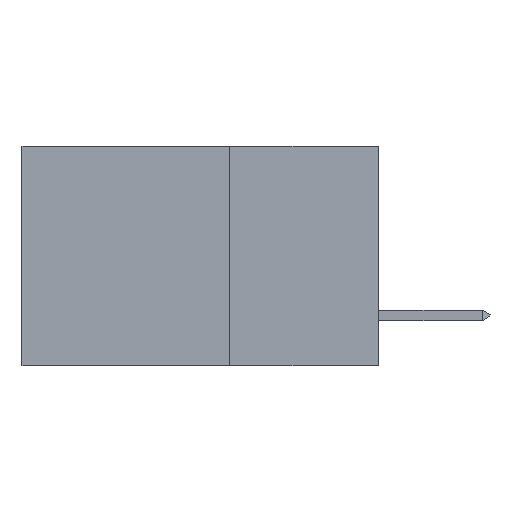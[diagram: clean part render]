
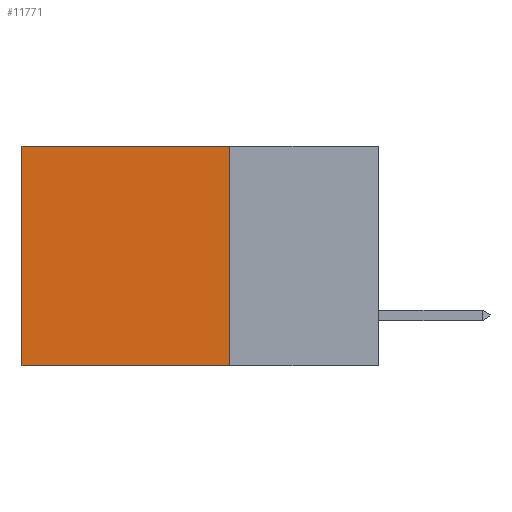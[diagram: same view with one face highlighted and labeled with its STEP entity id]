
A CAD part, left-side view. The second image highlights one B-rep face of the part: STEP entity #11771.
In plain terms, the highlighted planar face has unit normal (-1, 0, 0).
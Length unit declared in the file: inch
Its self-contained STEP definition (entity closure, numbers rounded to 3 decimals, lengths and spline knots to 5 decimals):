
#22 = VECTOR ( 'NONE', #3976, 39.37008 ) ;
#411 = EDGE_CURVE ( 'NONE', #11928, #7889, #801, .T. ) ;
#801 = LINE ( 'NONE', #11834, #3506 ) ;
#879 = EDGE_CURVE ( 'NONE', #6052, #7889, #10992, .T. ) ;
#984 = ORIENTED_EDGE ( 'NONE', *, *, #5597, .F. ) ;
#1007 = ORIENTED_EDGE ( 'NONE', *, *, #5497, .T. ) ;
#1047 = CARTESIAN_POINT ( 'NONE',  ( 0.298, 0.6, 0. ) ) ;
#1145 = DIRECTION ( 'NONE',  ( 0., 0., -1. ) ) ;
#1468 = DIRECTION ( 'NONE',  ( 0., 1., 0. ) ) ;
#1793 = CARTESIAN_POINT ( 'NONE',  ( 0.298, 0.25, 0. ) ) ;
#2299 = CARTESIAN_POINT ( 'NONE',  ( 0.298, 0.25, -0.37 ) ) ;
#3506 = VECTOR ( 'NONE', #1468, 39.37008 ) ;
#3549 = LINE ( 'NONE', #3564, #8967 ) ;
#3564 = CARTESIAN_POINT ( 'NONE',  ( 0.298, 0.25, 0. ) ) ;
#3764 = FACE_OUTER_BOUND ( 'NONE', #10693, .T. ) ;
#3894 = LINE ( 'NONE', #1793, #9603 ) ;
#3976 = DIRECTION ( 'NONE',  ( 0., 0., -1. ) ) ;
#4881 = PLANE ( 'NONE',  #5371 ) ;
#5371 = AXIS2_PLACEMENT_3D ( 'NONE', #9572, #10713, #7845 ) ;
#5497 = EDGE_CURVE ( 'NONE', #9509, #6052, #3549, .T. ) ;
#5597 = EDGE_CURVE ( 'NONE', #9509, #11928, #3894, .T. ) ;
#6052 = VERTEX_POINT ( 'NONE', #6452 ) ;
#6452 = CARTESIAN_POINT ( 'NONE',  ( 0.298, 0.6, 0. ) ) ;
#7845 = DIRECTION ( 'NONE',  ( 0., 0., -1. ) ) ;
#7889 = VERTEX_POINT ( 'NONE', #8202 ) ;
#8202 = CARTESIAN_POINT ( 'NONE',  ( 0.298, 0.6, -0.37 ) ) ;
#8967 = VECTOR ( 'NONE', #9343, 39.37008 ) ;
#9343 = DIRECTION ( 'NONE',  ( 0., 1., 0. ) ) ;
#9509 = VERTEX_POINT ( 'NONE', #9685 ) ;
#9572 = CARTESIAN_POINT ( 'NONE',  ( 0.298, 0.25, 0. ) ) ;
#9603 = VECTOR ( 'NONE', #1145, 39.37008 ) ;
#9683 = ORIENTED_EDGE ( 'NONE', *, *, #411, .F. ) ;
#9685 = CARTESIAN_POINT ( 'NONE',  ( 0.298, 0.25, 0. ) ) ;
#10489 = ORIENTED_EDGE ( 'NONE', *, *, #879, .T. ) ;
#10693 = EDGE_LOOP ( 'NONE', ( #10489, #9683, #984, #1007 ) ) ;
#10713 = DIRECTION ( 'NONE',  ( 1., 0., 0. ) ) ;
#10992 = LINE ( 'NONE', #1047, #22 ) ;
#11771 = ADVANCED_FACE ( 'NONE', ( #3764 ), #4881, .F. ) ;
#11834 = CARTESIAN_POINT ( 'NONE',  ( 0.298, 0.25, -0.37 ) ) ;
#11928 = VERTEX_POINT ( 'NONE', #2299 ) ;
